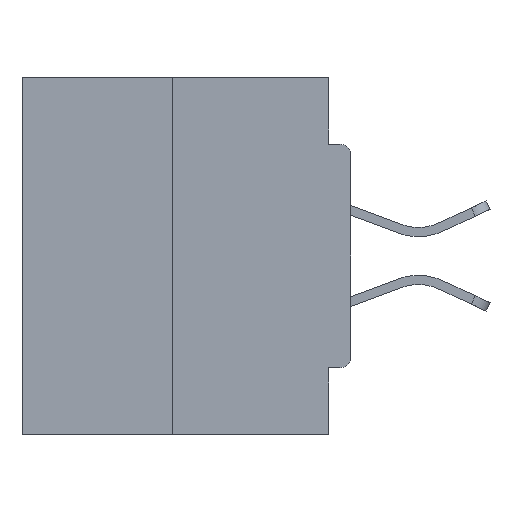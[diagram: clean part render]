
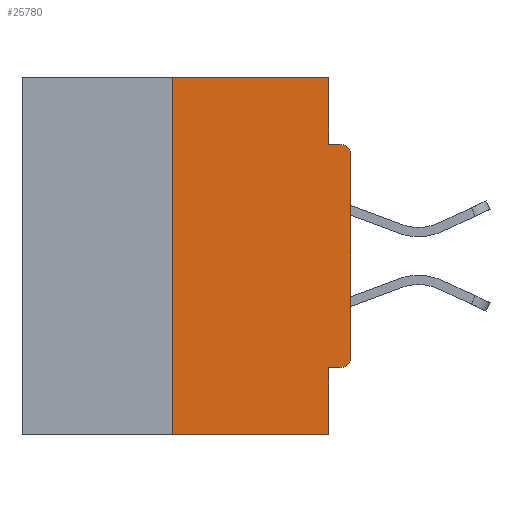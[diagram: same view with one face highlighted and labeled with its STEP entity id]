
A CAD part, left-side view. The second image highlights one B-rep face of the part: STEP entity #25780.
In plain terms, the highlighted planar face has unit normal (-1, 0, 0).
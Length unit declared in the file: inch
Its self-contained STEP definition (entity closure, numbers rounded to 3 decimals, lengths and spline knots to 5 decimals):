
#101 = EDGE_CURVE ( 'NONE', #36071, #10761, #5321, .T. ) ;
#429 = EDGE_LOOP ( 'NONE', ( #12342, #28359, #32768, #19288, #33433, #10224, #18493, #19599, #34920, #33068 ) ) ;
#764 = EDGE_CURVE ( 'NONE', #36071, #20169, #31399, .T. ) ;
#1355 = LINE ( 'NONE', #28638, #2209 ) ;
#2136 = VERTEX_POINT ( 'NONE', #10930 ) ;
#2209 = VECTOR ( 'NONE', #32043, 39.37008 ) ;
#2814 = CARTESIAN_POINT ( 'NONE',  ( 0., 0.031, -0.0935 ) ) ;
#3768 = CARTESIAN_POINT ( 'NONE',  ( 0., 0.015, -0.4065 ) ) ;
#5007 = VECTOR ( 'NONE', #31552, 39.37008 ) ;
#5321 = CIRCLE ( 'NONE', #26006, 0.015 ) ;
#5718 = CARTESIAN_POINT ( 'NONE',  ( 0., 0.015, -0.0935 ) ) ;
#6988 = DIRECTION ( 'NONE',  ( 0., -1., 0. ) ) ;
#8052 = LINE ( 'NONE', #28906, #9409 ) ;
#8468 = VERTEX_POINT ( 'NONE', #2814 ) ;
#8505 = DIRECTION ( 'NONE',  ( 1., 0., 0. ) ) ;
#8668 = EDGE_CURVE ( 'NONE', #2136, #8468, #20198, .T. ) ;
#8916 = AXIS2_PLACEMENT_3D ( 'NONE', #22079, #33236, #24973 ) ;
#9274 = CARTESIAN_POINT ( 'NONE',  ( 0., 0., -0.4065 ) ) ;
#9409 = VECTOR ( 'NONE', #20194, 39.37008 ) ;
#10224 = ORIENTED_EDGE ( 'NONE', *, *, #101, .T. ) ;
#10761 = VERTEX_POINT ( 'NONE', #21488 ) ;
#10930 = CARTESIAN_POINT ( 'NONE',  ( 0., 0.031, 0. ) ) ;
#11120 = EDGE_CURVE ( 'NONE', #20169, #22633, #31789, .T. ) ;
#11230 = VECTOR ( 'NONE', #35038, 39.37008 ) ;
#11417 = CARTESIAN_POINT ( 'NONE',  ( 0., 0.031, -0.4065 ) ) ;
#12342 = ORIENTED_EDGE ( 'NONE', *, *, #21185, .F. ) ;
#12634 = CARTESIAN_POINT ( 'NONE',  ( 0., 0.46, 0. ) ) ;
#13990 = CARTESIAN_POINT ( 'NONE',  ( 0., 0., -0.0935 ) ) ;
#15150 = VERTEX_POINT ( 'NONE', #31386 ) ;
#15528 = VECTOR ( 'NONE', #34750, 39.37008 ) ;
#16372 = EDGE_CURVE ( 'NONE', #10761, #17873, #8052, .T. ) ;
#16648 = DIRECTION ( 'NONE',  ( 0., 0., -1. ) ) ;
#17035 = PLANE ( 'NONE',  #20444 ) ;
#17553 = VECTOR ( 'NONE', #6988, 39.37008 ) ;
#17873 = VERTEX_POINT ( 'NONE', #25597 ) ;
#18493 = ORIENTED_EDGE ( 'NONE', *, *, #16372, .T. ) ;
#19288 = ORIENTED_EDGE ( 'NONE', *, *, #11120, .F. ) ;
#19599 = ORIENTED_EDGE ( 'NONE', *, *, #34405, .T. ) ;
#19849 = FACE_OUTER_BOUND ( 'NONE', #429, .T. ) ;
#20169 = VERTEX_POINT ( 'NONE', #11417 ) ;
#20194 = DIRECTION ( 'NONE',  ( 0., 0., 1. ) ) ;
#20198 = LINE ( 'NONE', #21250, #32384 ) ;
#20302 = LINE ( 'NONE', #13990, #5007 ) ;
#20444 = AXIS2_PLACEMENT_3D ( 'NONE', #25718, #8505, #16648 ) ;
#20803 = EDGE_CURVE ( 'NONE', #8468, #31228, #20302, .T. ) ;
#21185 = EDGE_CURVE ( 'NONE', #15150, #2136, #27035, .T. ) ;
#21250 = CARTESIAN_POINT ( 'NONE',  ( 0., 0.031, 0. ) ) ;
#21274 = VERTEX_POINT ( 'NONE', #33180 ) ;
#21488 = CARTESIAN_POINT ( 'NONE',  ( 0., 0., -0.3915 ) ) ;
#21626 = CARTESIAN_POINT ( 'NONE',  ( 0., 0.031, -0.5 ) ) ;
#22079 = CARTESIAN_POINT ( 'NONE',  ( 0., 0.015, -0.1085 ) ) ;
#22633 = VERTEX_POINT ( 'NONE', #21626 ) ;
#23005 = CARTESIAN_POINT ( 'NONE',  ( 0., 0.015, -0.3915 ) ) ;
#23622 = CARTESIAN_POINT ( 'NONE',  ( 0., 0.25, 0. ) ) ;
#24156 = VECTOR ( 'NONE', #32223, 39.37008 ) ;
#24973 = DIRECTION ( 'NONE',  ( 0., 0., -1. ) ) ;
#25597 = CARTESIAN_POINT ( 'NONE',  ( 0., 0., -0.1085 ) ) ;
#25718 = CARTESIAN_POINT ( 'NONE',  ( 0., 0.46, 0. ) ) ;
#25780 = ADVANCED_FACE ( 'NONE', ( #19849 ), #17035, .F. ) ;
#25862 = CARTESIAN_POINT ( 'NONE',  ( 0., 0.031, -0.5 ) ) ;
#26006 = AXIS2_PLACEMENT_3D ( 'NONE', #23005, #34299, #31499 ) ;
#26563 = LINE ( 'NONE', #23622, #11230 ) ;
#27035 = LINE ( 'NONE', #12634, #17553 ) ;
#27410 = EDGE_CURVE ( 'NONE', #21274, #22633, #1355, .T. ) ;
#28359 = ORIENTED_EDGE ( 'NONE', *, *, #34959, .F. ) ;
#28638 = CARTESIAN_POINT ( 'NONE',  ( 0., 0.46, -0.5 ) ) ;
#28906 = CARTESIAN_POINT ( 'NONE',  ( 0., 0., 0. ) ) ;
#30106 = DIRECTION ( 'NONE',  ( 0., 0., -1. ) ) ;
#30648 = CIRCLE ( 'NONE', #8916, 0.015 ) ;
#31228 = VERTEX_POINT ( 'NONE', #5718 ) ;
#31386 = CARTESIAN_POINT ( 'NONE',  ( 0., 0.25, 0. ) ) ;
#31399 = LINE ( 'NONE', #9274, #24156 ) ;
#31499 = DIRECTION ( 'NONE',  ( 0., 0., -1. ) ) ;
#31552 = DIRECTION ( 'NONE',  ( 0., -1., 0. ) ) ;
#31789 = LINE ( 'NONE', #25862, #15528 ) ;
#32043 = DIRECTION ( 'NONE',  ( 0., -1., 0. ) ) ;
#32223 = DIRECTION ( 'NONE',  ( 0., 1., 0. ) ) ;
#32384 = VECTOR ( 'NONE', #30106, 39.37008 ) ;
#32768 = ORIENTED_EDGE ( 'NONE', *, *, #27410, .T. ) ;
#33068 = ORIENTED_EDGE ( 'NONE', *, *, #8668, .F. ) ;
#33180 = CARTESIAN_POINT ( 'NONE',  ( 0., 0.25, -0.5 ) ) ;
#33236 = DIRECTION ( 'NONE',  ( -1., 0., 0. ) ) ;
#33433 = ORIENTED_EDGE ( 'NONE', *, *, #764, .F. ) ;
#34299 = DIRECTION ( 'NONE',  ( -1., 0., 0. ) ) ;
#34405 = EDGE_CURVE ( 'NONE', #17873, #31228, #30648, .T. ) ;
#34750 = DIRECTION ( 'NONE',  ( 0., 0., -1. ) ) ;
#34920 = ORIENTED_EDGE ( 'NONE', *, *, #20803, .F. ) ;
#34959 = EDGE_CURVE ( 'NONE', #21274, #15150, #26563, .T. ) ;
#35038 = DIRECTION ( 'NONE',  ( 0., 0., 1. ) ) ;
#36071 = VERTEX_POINT ( 'NONE', #3768 ) ;
